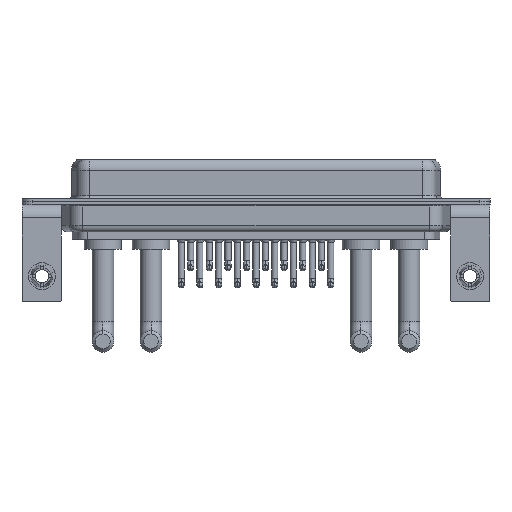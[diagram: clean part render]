
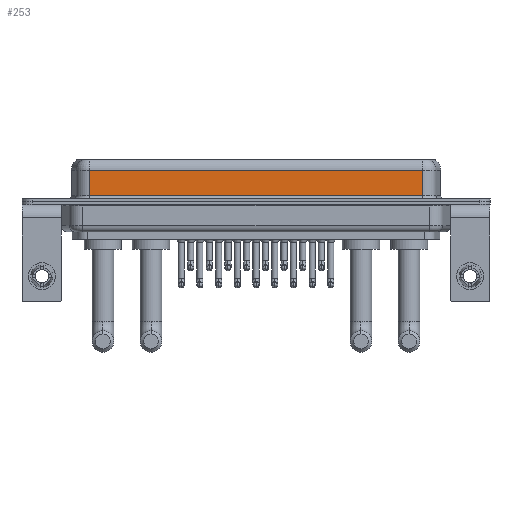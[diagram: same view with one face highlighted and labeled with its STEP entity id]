
A CAD part, front view. The second image highlights one B-rep face of the part: STEP entity #253.
In plain terms, the highlighted planar face has unit normal (0, -1, 0).
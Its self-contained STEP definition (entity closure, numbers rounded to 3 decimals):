
#253 = ADVANCED_FACE ( 'NONE', ( #13686 ), #19110, .F. ) ;
#1259 = DIRECTION ( 'NONE',  ( -1., 0., 0. ) ) ;
#1446 = VERTEX_POINT ( 'NONE', #10234 ) ;
#1513 = LINE ( 'NONE', #9062, #4406 ) ;
#2187 = DIRECTION ( 'NONE',  ( 0., 1., 0. ) ) ;
#3179 = VECTOR ( 'NONE', #3384, 1000. ) ;
#3384 = DIRECTION ( 'NONE',  ( 1., 0., 0. ) ) ;
#3503 = ORIENTED_EDGE ( 'NONE', *, *, #20679, .F. ) ;
#4406 = VECTOR ( 'NONE', #9301, 1000. ) ;
#6648 = CARTESIAN_POINT ( 'NONE',  ( 7.038, -3.95, 4.65 ) ) ;
#6810 = EDGE_CURVE ( 'NONE', #1446, #24394, #14636, .T. ) ;
#6884 = ORIENTED_EDGE ( 'NONE', *, *, #6810, .T. ) ;
#8615 = EDGE_LOOP ( 'NONE', ( #3503, #10299, #23497, #6884 ) ) ;
#8697 = VECTOR ( 'NONE', #1259, 1000. ) ;
#9062 = CARTESIAN_POINT ( 'NONE',  ( 56.462, -3.95, 6.4 ) ) ;
#9301 = DIRECTION ( 'NONE',  ( 0., 0., -1. ) ) ;
#9728 = CARTESIAN_POINT ( 'NONE',  ( 56.462, -3.95, 0.9 ) ) ;
#9810 = CARTESIAN_POINT ( 'NONE',  ( 7.038, -3.95, 6.4 ) ) ;
#10234 = CARTESIAN_POINT ( 'NONE',  ( 7.038, -3.95, 0.9 ) ) ;
#10299 = ORIENTED_EDGE ( 'NONE', *, *, #16044, .T. ) ;
#10760 = LINE ( 'NONE', #18635, #8697 ) ;
#10985 = EDGE_CURVE ( 'NONE', #15077, #1446, #17334, .T. ) ;
#11887 = CARTESIAN_POINT ( 'NONE',  ( 56.462, -3.95, 4.65 ) ) ;
#13686 = FACE_OUTER_BOUND ( 'NONE', #8615, .T. ) ;
#14636 = LINE ( 'NONE', #16122, #3179 ) ;
#15077 = VERTEX_POINT ( 'NONE', #6648 ) ;
#15545 = CARTESIAN_POINT ( 'NONE',  ( 56.462, -3.95, 6.4 ) ) ;
#15855 = VERTEX_POINT ( 'NONE', #11887 ) ;
#16044 = EDGE_CURVE ( 'NONE', #15855, #15077, #10760, .T. ) ;
#16122 = CARTESIAN_POINT ( 'NONE',  ( 56.462, -3.95, 0.9 ) ) ;
#16184 = VECTOR ( 'NONE', #19314, 1000. ) ;
#16896 = DIRECTION ( 'NONE',  ( 0., 0., 1. ) ) ;
#17334 = LINE ( 'NONE', #9810, #16184 ) ;
#18635 = CARTESIAN_POINT ( 'NONE',  ( 56.462, -3.95, 4.65 ) ) ;
#19110 = PLANE ( 'NONE',  #22847 ) ;
#19314 = DIRECTION ( 'NONE',  ( 0., 0., -1. ) ) ;
#20679 = EDGE_CURVE ( 'NONE', #15855, #24394, #1513, .T. ) ;
#22847 = AXIS2_PLACEMENT_3D ( 'NONE', #15545, #2187, #16896 ) ;
#23497 = ORIENTED_EDGE ( 'NONE', *, *, #10985, .T. ) ;
#24394 = VERTEX_POINT ( 'NONE', #9728 ) ;
